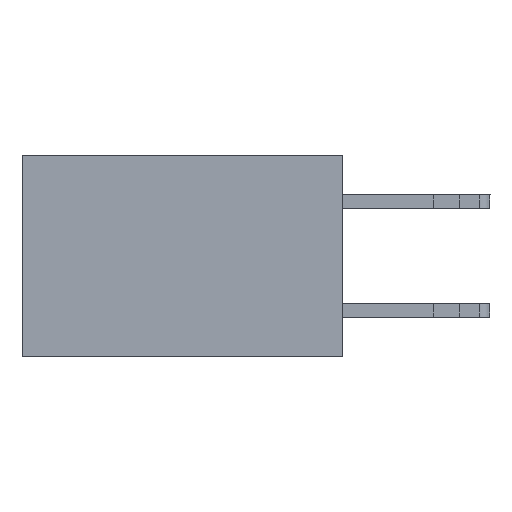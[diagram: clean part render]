
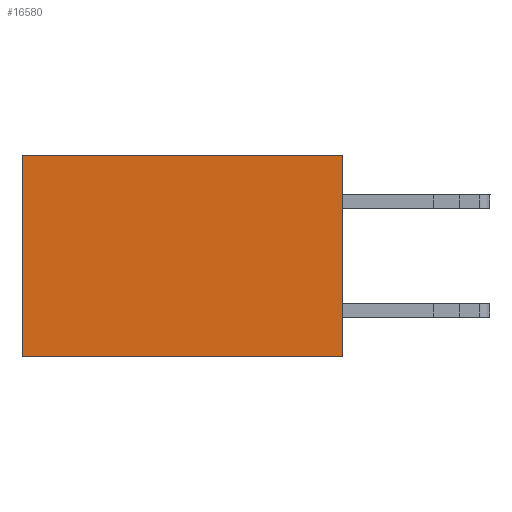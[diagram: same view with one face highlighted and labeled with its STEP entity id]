
A CAD part, left-side view. The second image highlights one B-rep face of the part: STEP entity #16580.
In plain terms, the highlighted planar face has unit normal (-1, 0, 0).
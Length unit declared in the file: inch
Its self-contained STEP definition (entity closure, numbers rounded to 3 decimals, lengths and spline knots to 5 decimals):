
#458 = LINE ( 'NONE', #20226, #17023 ) ;
#1338 = DIRECTION ( 'NONE',  ( 0., 1., 0. ) ) ;
#1941 = ORIENTED_EDGE ( 'NONE', *, *, #8481, .F. ) ;
#3296 = VERTEX_POINT ( 'NONE', #6093 ) ;
#3604 = CARTESIAN_POINT ( 'NONE',  ( 0.277, 0., -0.37 ) ) ;
#3658 = VECTOR ( 'NONE', #9158, 39.37008 ) ;
#3755 = CARTESIAN_POINT ( 'NONE',  ( 0.277, 0., -0.37 ) ) ;
#3827 = ORIENTED_EDGE ( 'NONE', *, *, #17387, .T. ) ;
#4521 = CARTESIAN_POINT ( 'NONE',  ( 0.277, 0., -0.37 ) ) ;
#4714 = CARTESIAN_POINT ( 'NONE',  ( 0.277, 0.59, 0. ) ) ;
#5151 = DIRECTION ( 'NONE',  ( 0., 0., -1. ) ) ;
#5307 = ORIENTED_EDGE ( 'NONE', *, *, #11314, .T. ) ;
#5385 = DIRECTION ( 'NONE',  ( 0., 0., -1. ) ) ;
#5422 = PLANE ( 'NONE',  #6656 ) ;
#6093 = CARTESIAN_POINT ( 'NONE',  ( 0.277, 0.59, -0.37 ) ) ;
#6656 = AXIS2_PLACEMENT_3D ( 'NONE', #12600, #19204, #20711 ) ;
#7019 = EDGE_LOOP ( 'NONE', ( #3827, #17983, #1941, #5307 ) ) ;
#7299 = LINE ( 'NONE', #7416, #3658 ) ;
#7416 = CARTESIAN_POINT ( 'NONE',  ( 0.277, 0., 0. ) ) ;
#8481 = EDGE_CURVE ( 'NONE', #10106, #15868, #13975, .T. ) ;
#9158 = DIRECTION ( 'NONE',  ( 0., 1., 0. ) ) ;
#10106 = VERTEX_POINT ( 'NONE', #16689 ) ;
#11164 = VECTOR ( 'NONE', #1338, 39.37008 ) ;
#11314 = EDGE_CURVE ( 'NONE', #10106, #20528, #7299, .T. ) ;
#12600 = CARTESIAN_POINT ( 'NONE',  ( 0.277, 0., -0.37 ) ) ;
#12675 = LINE ( 'NONE', #4521, #11164 ) ;
#13975 = LINE ( 'NONE', #3755, #15285 ) ;
#15285 = VECTOR ( 'NONE', #5385, 39.37008 ) ;
#15868 = VERTEX_POINT ( 'NONE', #3604 ) ;
#16580 = ADVANCED_FACE ( 'NONE', ( #20279 ), #5422, .F. ) ;
#16689 = CARTESIAN_POINT ( 'NONE',  ( 0.277, 0., 0. ) ) ;
#17023 = VECTOR ( 'NONE', #5151, 39.37008 ) ;
#17387 = EDGE_CURVE ( 'NONE', #20528, #3296, #458, .T. ) ;
#17983 = ORIENTED_EDGE ( 'NONE', *, *, #18397, .F. ) ;
#18397 = EDGE_CURVE ( 'NONE', #15868, #3296, #12675, .T. ) ;
#19204 = DIRECTION ( 'NONE',  ( 1., 0., 0. ) ) ;
#20226 = CARTESIAN_POINT ( 'NONE',  ( 0.277, 0.59, -0.37 ) ) ;
#20279 = FACE_OUTER_BOUND ( 'NONE', #7019, .T. ) ;
#20528 = VERTEX_POINT ( 'NONE', #4714 ) ;
#20711 = DIRECTION ( 'NONE',  ( 0., 0., -1. ) ) ;
